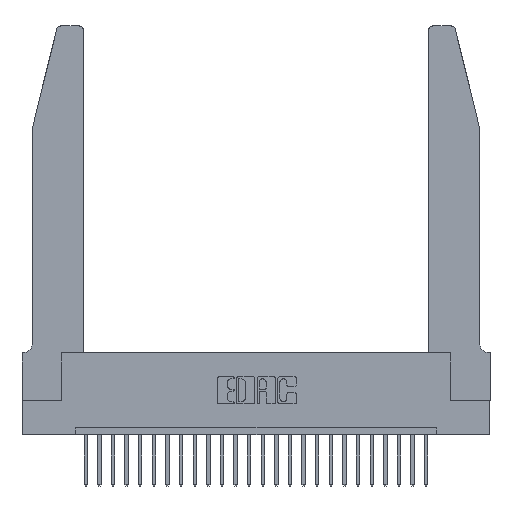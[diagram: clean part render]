
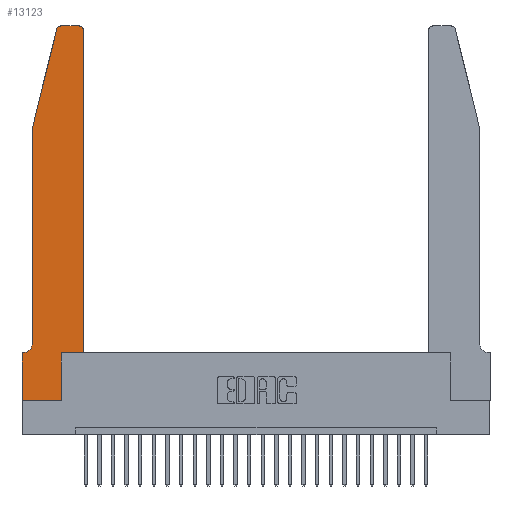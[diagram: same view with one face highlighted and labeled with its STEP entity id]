
A CAD part, top view. The second image highlights one B-rep face of the part: STEP entity #13123.
In plain terms, the highlighted planar face has unit normal (0, 0, 1).
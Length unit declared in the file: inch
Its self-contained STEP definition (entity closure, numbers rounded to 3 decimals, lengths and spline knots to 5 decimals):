
#5 = ORIENTED_EDGE ( 'NONE', *, *, #21902, .T. ) ;
#9 = VERTEX_POINT ( 'NONE', #7524 ) ;
#111 = VERTEX_POINT ( 'NONE', #6794 ) ;
#142 = CARTESIAN_POINT ( 'NONE',  ( 0., 0.35, 0.37 ) ) ;
#246 = ORIENTED_EDGE ( 'NONE', *, *, #5877, .T. ) ;
#376 = DIRECTION ( 'NONE',  ( -0.239, -0.971, 0. ) ) ;
#443 = DIRECTION ( 'NONE',  ( 1., 0., 0. ) ) ;
#519 = EDGE_CURVE ( 'NONE', #11558, #2911, #3962, .T. ) ;
#559 = VECTOR ( 'NONE', #25499, 39.37008 ) ;
#686 = ORIENTED_EDGE ( 'NONE', *, *, #5314, .T. ) ;
#1411 = ORIENTED_EDGE ( 'NONE', *, *, #20811, .T. ) ;
#1698 = LINE ( 'NONE', #6885, #19329 ) ;
#2166 = CARTESIAN_POINT ( 'NONE',  ( 0.4505, 0.35, 0.37 ) ) ;
#2280 = DIRECTION ( 'NONE',  ( 1., 0., 0. ) ) ;
#2317 = DIRECTION ( 'NONE',  ( 0., 1., 0. ) ) ;
#2491 = VERTEX_POINT ( 'NONE', #13245 ) ;
#2510 = CARTESIAN_POINT ( 'NONE',  ( 0.2865, 0.35, 0.37 ) ) ;
#2911 = VERTEX_POINT ( 'NONE', #16606 ) ;
#3038 = DIRECTION ( 'NONE',  ( 0., -1., 0. ) ) ;
#3077 = CIRCLE ( 'NONE', #3281, 0.07 ) ;
#3268 = LINE ( 'NONE', #6043, #12835 ) ;
#3281 = AXIS2_PLACEMENT_3D ( 'NONE', #11563, #21667, #23716 ) ;
#3295 = ORIENTED_EDGE ( 'NONE', *, *, #519, .T. ) ;
#3875 = EDGE_CURVE ( 'NONE', #19236, #3888, #12303, .T. ) ;
#3888 = VERTEX_POINT ( 'NONE', #15439 ) ;
#3962 = LINE ( 'NONE', #12555, #10662 ) ;
#4392 = EDGE_CURVE ( 'NONE', #11448, #11558, #8748, .T. ) ;
#4489 = DIRECTION ( 'NONE',  ( 0., 1., 0. ) ) ;
#4646 = VECTOR ( 'NONE', #16781, 39.37008 ) ;
#4913 = DIRECTION ( 'NONE',  ( -1., 0., 0. ) ) ;
#5314 = EDGE_CURVE ( 'NONE', #21327, #25133, #7732, .T. ) ;
#5546 = LINE ( 'NONE', #25623, #9409 ) ;
#5877 = EDGE_CURVE ( 'NONE', #2911, #19236, #9014, .T. ) ;
#6043 = CARTESIAN_POINT ( 'NONE',  ( 0.0755, 2., 0.37 ) ) ;
#6794 = CARTESIAN_POINT ( 'NONE',  ( 0.25487, 2.72718, 0.37 ) ) ;
#6885 = CARTESIAN_POINT ( 'NONE',  ( 0., 0., 0.37 ) ) ;
#7524 = CARTESIAN_POINT ( 'NONE',  ( 0.0755, 0.42, 0.37 ) ) ;
#7732 = LINE ( 'NONE', #23196, #14474 ) ;
#8592 = CARTESIAN_POINT ( 'NONE',  ( 0.284, 2.72, 0.37 ) ) ;
#8748 = LINE ( 'NONE', #2166, #4646 ) ;
#9014 = CIRCLE ( 'NONE', #10609, 0.03 ) ;
#9409 = VECTOR ( 'NONE', #13622, 39.37008 ) ;
#9445 = ORIENTED_EDGE ( 'NONE', *, *, #4392, .T. ) ;
#9904 = VERTEX_POINT ( 'NONE', #22072 ) ;
#10292 = ORIENTED_EDGE ( 'NONE', *, *, #26178, .T. ) ;
#10307 = ORIENTED_EDGE ( 'NONE', *, *, #22325, .T. ) ;
#10609 = AXIS2_PLACEMENT_3D ( 'NONE', #12747, #14546, #2280 ) ;
#10662 = VECTOR ( 'NONE', #4489, 39.37008 ) ;
#11448 = VERTEX_POINT ( 'NONE', #16395 ) ;
#11558 = VERTEX_POINT ( 'NONE', #25588 ) ;
#11563 = CARTESIAN_POINT ( 'NONE',  ( 0.0055, 0.42, 0.37 ) ) ;
#11702 = ORIENTED_EDGE ( 'NONE', *, *, #3875, .T. ) ;
#11919 = EDGE_CURVE ( 'NONE', #9904, #9, #5546, .T. ) ;
#11921 = CIRCLE ( 'NONE', #20601, 0.03 ) ;
#12172 = DIRECTION ( 'NONE',  ( 0., 0., 1. ) ) ;
#12303 = LINE ( 'NONE', #19428, #13600 ) ;
#12555 = CARTESIAN_POINT ( 'NONE',  ( 0.4505, 0.35, 0.37 ) ) ;
#12747 = CARTESIAN_POINT ( 'NONE',  ( 0.4205, 2.72, 0.37 ) ) ;
#12835 = VECTOR ( 'NONE', #376, 39.37008 ) ;
#13123 = ADVANCED_FACE ( 'NONE', ( #15424 ), #15846, .T. ) ;
#13245 = CARTESIAN_POINT ( 'NONE',  ( 0., 0., 0.37 ) ) ;
#13452 = CARTESIAN_POINT ( 'NONE',  ( 0., 0.35, 0.37 ) ) ;
#13600 = VECTOR ( 'NONE', #21942, 39.37008 ) ;
#13622 = DIRECTION ( 'NONE',  ( 0., -1., 0. ) ) ;
#14094 = VECTOR ( 'NONE', #2317, 39.37008 ) ;
#14322 = DIRECTION ( 'NONE',  ( 1., 0., 0. ) ) ;
#14474 = VECTOR ( 'NONE', #4913, 39.37008 ) ;
#14546 = DIRECTION ( 'NONE',  ( 0., 0., 1. ) ) ;
#14646 = CARTESIAN_POINT ( 'NONE',  ( 0.0055, 0.35, 0.37 ) ) ;
#15033 = ORIENTED_EDGE ( 'NONE', *, *, #11919, .T. ) ;
#15424 = FACE_OUTER_BOUND ( 'NONE', #16118, .T. ) ;
#15439 = CARTESIAN_POINT ( 'NONE',  ( 0.284, 2.75, 0.37 ) ) ;
#15846 = PLANE ( 'NONE',  #21350 ) ;
#15903 = CARTESIAN_POINT ( 'NONE',  ( 0.4205, 2.75, 0.37 ) ) ;
#16118 = EDGE_LOOP ( 'NONE', ( #11702, #1411, #5, #15033, #25553, #686, #10292, #16446, #10307, #9445, #3295, #246 ) ) ;
#16395 = CARTESIAN_POINT ( 'NONE',  ( 0.2865, 0.35, 0.37 ) ) ;
#16446 = ORIENTED_EDGE ( 'NONE', *, *, #24033, .T. ) ;
#16606 = CARTESIAN_POINT ( 'NONE',  ( 0.4505, 2.72, 0.37 ) ) ;
#16691 = VERTEX_POINT ( 'NONE', #26345 ) ;
#16781 = DIRECTION ( 'NONE',  ( 1., 0., 0. ) ) ;
#16840 = DIRECTION ( 'NONE',  ( 0., 0., 1. ) ) ;
#17559 = EDGE_CURVE ( 'NONE', #9, #21327, #3077, .T. ) ;
#19236 = VERTEX_POINT ( 'NONE', #15903 ) ;
#19329 = VECTOR ( 'NONE', #3038, 39.37008 ) ;
#19428 = CARTESIAN_POINT ( 'NONE',  ( 0.2605, 2.75, 0.37 ) ) ;
#20601 = AXIS2_PLACEMENT_3D ( 'NONE', #8592, #16840, #443 ) ;
#20811 = EDGE_CURVE ( 'NONE', #3888, #111, #11921, .T. ) ;
#21327 = VERTEX_POINT ( 'NONE', #14646 ) ;
#21350 = AXIS2_PLACEMENT_3D ( 'NONE', #142, #12172, #14322 ) ;
#21667 = DIRECTION ( 'NONE',  ( 0., 0., -1. ) ) ;
#21902 = EDGE_CURVE ( 'NONE', #111, #9904, #3268, .T. ) ;
#21942 = DIRECTION ( 'NONE',  ( -1., 0., 0. ) ) ;
#22072 = CARTESIAN_POINT ( 'NONE',  ( 0.0755, 2., 0.37 ) ) ;
#22325 = EDGE_CURVE ( 'NONE', #16691, #11448, #25292, .T. ) ;
#23196 = CARTESIAN_POINT ( 'NONE',  ( 0.0755, 0.35, 0.37 ) ) ;
#23439 = CARTESIAN_POINT ( 'NONE',  ( 0., 0., 0.37 ) ) ;
#23716 = DIRECTION ( 'NONE',  ( -1., 0., 0. ) ) ;
#24033 = EDGE_CURVE ( 'NONE', #2491, #16691, #26466, .T. ) ;
#25133 = VERTEX_POINT ( 'NONE', #13452 ) ;
#25292 = LINE ( 'NONE', #2510, #14094 ) ;
#25499 = DIRECTION ( 'NONE',  ( 1., 0., 0. ) ) ;
#25553 = ORIENTED_EDGE ( 'NONE', *, *, #17559, .T. ) ;
#25588 = CARTESIAN_POINT ( 'NONE',  ( 0.4505, 0.35, 0.37 ) ) ;
#25623 = CARTESIAN_POINT ( 'NONE',  ( 0.0755, 2., 0.37 ) ) ;
#26178 = EDGE_CURVE ( 'NONE', #25133, #2491, #1698, .T. ) ;
#26345 = CARTESIAN_POINT ( 'NONE',  ( 0.2865, 0., 0.37 ) ) ;
#26466 = LINE ( 'NONE', #23439, #559 ) ;
